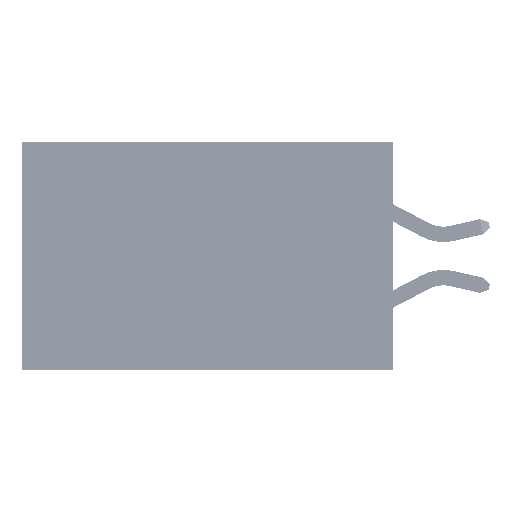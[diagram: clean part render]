
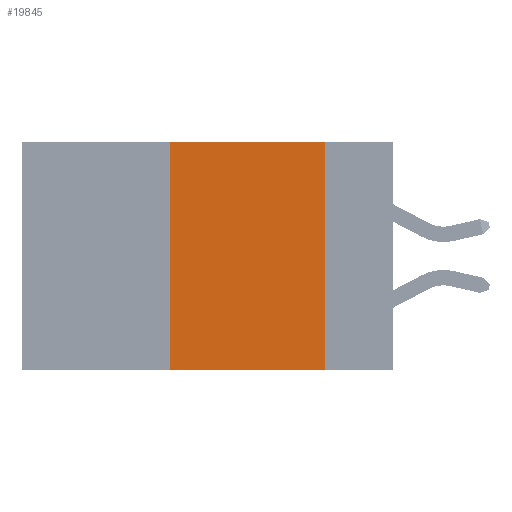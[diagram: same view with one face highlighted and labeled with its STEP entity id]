
A CAD part, left-side view. The second image highlights one B-rep face of the part: STEP entity #19845.
In plain terms, the highlighted planar face has unit normal (-1, 0, 0).
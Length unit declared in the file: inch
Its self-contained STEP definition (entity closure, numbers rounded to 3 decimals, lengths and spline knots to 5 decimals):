
#3334 = ORIENTED_EDGE ( 'NONE', *, *, #3597, .F. ) ;
#3597 = EDGE_CURVE ( 'NONE', #42181, #41116, #22943, .T. ) ;
#3750 = EDGE_LOOP ( 'NONE', ( #36050, #21304, #3334, #31994 ) ) ;
#6068 = CARTESIAN_POINT ( 'NONE',  ( 0., 0.6, 0. ) ) ;
#7304 = LINE ( 'NONE', #25051, #45247 ) ;
#7388 = VECTOR ( 'NONE', #15733, 39.37008 ) ;
#9975 = CARTESIAN_POINT ( 'NONE',  ( 0., 0.36, 0. ) ) ;
#10304 = VECTOR ( 'NONE', #40845, 39.37008 ) ;
#12869 = VERTEX_POINT ( 'NONE', #24730 ) ;
#15733 = DIRECTION ( 'NONE',  ( 0., 0., 1. ) ) ;
#15891 = CARTESIAN_POINT ( 'NONE',  ( 0., 0.36, 0. ) ) ;
#15983 = EDGE_CURVE ( 'NONE', #42181, #12869, #34196, .T. ) ;
#16472 = DIRECTION ( 'NONE',  ( 1., 0., 0. ) ) ;
#19000 = CARTESIAN_POINT ( 'NONE',  ( 0., 0.11, 0. ) ) ;
#19845 = ADVANCED_FACE ( 'NONE', ( #33198 ), #34328, .F. ) ;
#21304 = ORIENTED_EDGE ( 'NONE', *, *, #37918, .F. ) ;
#22943 = LINE ( 'NONE', #15891, #7388 ) ;
#23111 = AXIS2_PLACEMENT_3D ( 'NONE', #6068, #16472, #28201 ) ;
#24730 = CARTESIAN_POINT ( 'NONE',  ( 0., 0.11, -0.37 ) ) ;
#25004 = VECTOR ( 'NONE', #40719, 39.37008 ) ;
#25051 = CARTESIAN_POINT ( 'NONE',  ( 0., 0.6, 0. ) ) ;
#25424 = EDGE_CURVE ( 'NONE', #42941, #12869, #28132, .T. ) ;
#26591 = CARTESIAN_POINT ( 'NONE',  ( 0., 0.6, -0.37 ) ) ;
#28132 = LINE ( 'NONE', #19000, #10304 ) ;
#28201 = DIRECTION ( 'NONE',  ( 0., 0., -1. ) ) ;
#31091 = CARTESIAN_POINT ( 'NONE',  ( 0., 0.11, 0. ) ) ;
#31994 = ORIENTED_EDGE ( 'NONE', *, *, #15983, .T. ) ;
#32783 = CARTESIAN_POINT ( 'NONE',  ( 0., 0.36, -0.37 ) ) ;
#33198 = FACE_OUTER_BOUND ( 'NONE', #3750, .T. ) ;
#34196 = LINE ( 'NONE', #26591, #25004 ) ;
#34328 = PLANE ( 'NONE',  #23111 ) ;
#35850 = DIRECTION ( 'NONE',  ( 0., -1., 0. ) ) ;
#36050 = ORIENTED_EDGE ( 'NONE', *, *, #25424, .F. ) ;
#37918 = EDGE_CURVE ( 'NONE', #41116, #42941, #7304, .T. ) ;
#40719 = DIRECTION ( 'NONE',  ( 0., -1., 0. ) ) ;
#40845 = DIRECTION ( 'NONE',  ( 0., 0., -1. ) ) ;
#41116 = VERTEX_POINT ( 'NONE', #9975 ) ;
#42181 = VERTEX_POINT ( 'NONE', #32783 ) ;
#42941 = VERTEX_POINT ( 'NONE', #31091 ) ;
#45247 = VECTOR ( 'NONE', #35850, 39.37008 ) ;
